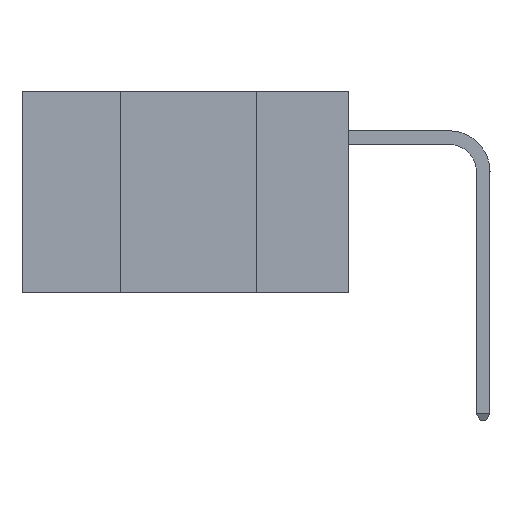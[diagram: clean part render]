
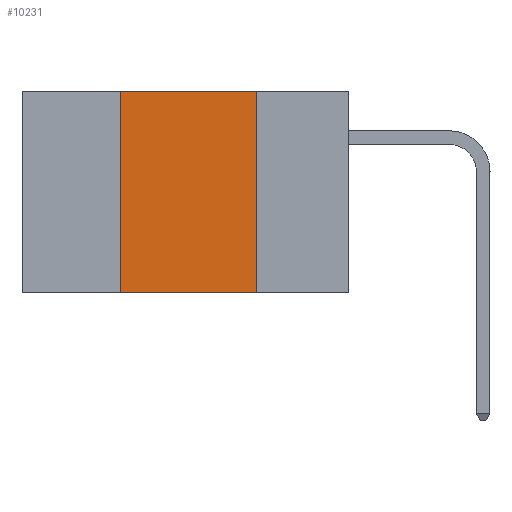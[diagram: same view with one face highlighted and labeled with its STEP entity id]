
A CAD part, left-side view. The second image highlights one B-rep face of the part: STEP entity #10231.
In plain terms, the highlighted planar face has unit normal (-1, 0, 0).
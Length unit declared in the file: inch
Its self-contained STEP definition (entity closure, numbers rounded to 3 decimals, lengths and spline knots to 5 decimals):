
#93 = VERTEX_POINT ( 'NONE', #7000 ) ;
#444 = LINE ( 'NONE', #7860, #13049 ) ;
#614 = CARTESIAN_POINT ( 'NONE',  ( 0., 0.6, 0. ) ) ;
#851 = FACE_OUTER_BOUND ( 'NONE', #2253, .T. ) ;
#2122 = CARTESIAN_POINT ( 'NONE',  ( 0., 0.42, 0. ) ) ;
#2253 = EDGE_LOOP ( 'NONE', ( #17675, #12522, #4513, #5836 ) ) ;
#3122 = DIRECTION ( 'NONE',  ( 0., -1., 0. ) ) ;
#3478 = DIRECTION ( 'NONE',  ( 0., -1., 0. ) ) ;
#3550 = DIRECTION ( 'NONE',  ( 1., 0., 0. ) ) ;
#3991 = DIRECTION ( 'NONE',  ( 0., 0., -1. ) ) ;
#4328 = AXIS2_PLACEMENT_3D ( 'NONE', #614, #3550, #6476 ) ;
#4513 = ORIENTED_EDGE ( 'NONE', *, *, #15063, .F. ) ;
#5195 = EDGE_CURVE ( 'NONE', #17814, #93, #444, .T. ) ;
#5836 = ORIENTED_EDGE ( 'NONE', *, *, #5195, .T. ) ;
#6336 = LINE ( 'NONE', #10819, #9191 ) ;
#6476 = DIRECTION ( 'NONE',  ( 0., 0., -1. ) ) ;
#6801 = PLANE ( 'NONE',  #4328 ) ;
#7000 = CARTESIAN_POINT ( 'NONE',  ( 0., 0.17, -0.37 ) ) ;
#7860 = CARTESIAN_POINT ( 'NONE',  ( 0., 0.6, -0.37 ) ) ;
#8575 = CARTESIAN_POINT ( 'NONE',  ( 0., 0.17, 0. ) ) ;
#8773 = LINE ( 'NONE', #8575, #11909 ) ;
#9191 = VECTOR ( 'NONE', #3122, 39.37008 ) ;
#9396 = CARTESIAN_POINT ( 'NONE',  ( 0., 0.42, 0. ) ) ;
#10231 = ADVANCED_FACE ( 'NONE', ( #851 ), #6801, .F. ) ;
#10819 = CARTESIAN_POINT ( 'NONE',  ( 0., 0.6, 0. ) ) ;
#11880 = VECTOR ( 'NONE', #15878, 39.37008 ) ;
#11909 = VECTOR ( 'NONE', #3991, 39.37008 ) ;
#12522 = ORIENTED_EDGE ( 'NONE', *, *, #18706, .F. ) ;
#13049 = VECTOR ( 'NONE', #3478, 39.37008 ) ;
#14346 = CARTESIAN_POINT ( 'NONE',  ( 0., 0.42, -0.37 ) ) ;
#14711 = CARTESIAN_POINT ( 'NONE',  ( 0., 0.17, 0. ) ) ;
#15063 = EDGE_CURVE ( 'NONE', #17814, #15922, #15490, .T. ) ;
#15490 = LINE ( 'NONE', #2122, #11880 ) ;
#15878 = DIRECTION ( 'NONE',  ( 0., 0., 1. ) ) ;
#15922 = VERTEX_POINT ( 'NONE', #9396 ) ;
#16007 = EDGE_CURVE ( 'NONE', #19026, #93, #8773, .T. ) ;
#17675 = ORIENTED_EDGE ( 'NONE', *, *, #16007, .F. ) ;
#17814 = VERTEX_POINT ( 'NONE', #14346 ) ;
#18706 = EDGE_CURVE ( 'NONE', #15922, #19026, #6336, .T. ) ;
#19026 = VERTEX_POINT ( 'NONE', #14711 ) ;
